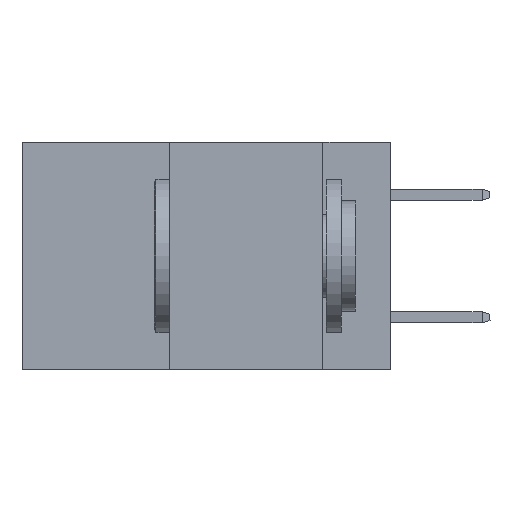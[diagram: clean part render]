
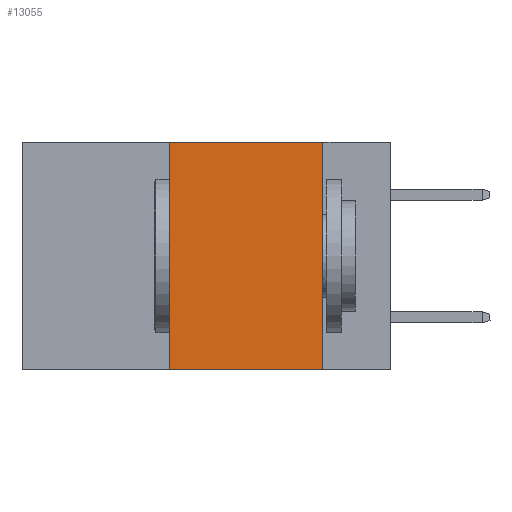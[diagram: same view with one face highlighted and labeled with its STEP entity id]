
A CAD part, left-side view. The second image highlights one B-rep face of the part: STEP entity #13055.
In plain terms, the highlighted planar face has unit normal (-1, 0, 0).
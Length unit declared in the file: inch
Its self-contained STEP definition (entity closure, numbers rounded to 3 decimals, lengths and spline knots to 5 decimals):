
#154 = LINE ( 'NONE', #2120, #3771 ) ;
#176 = DIRECTION ( 'NONE',  ( 0., 0., -1. ) ) ;
#605 = VERTEX_POINT ( 'NONE', #15817 ) ;
#864 = VECTOR ( 'NONE', #176, 39.37008 ) ;
#1067 = VERTEX_POINT ( 'NONE', #2170 ) ;
#2120 = CARTESIAN_POINT ( 'NONE',  ( 0., 0.6, 0. ) ) ;
#2170 = CARTESIAN_POINT ( 'NONE',  ( 0., 0.11, -0.37 ) ) ;
#2599 = VERTEX_POINT ( 'NONE', #12426 ) ;
#2916 = CARTESIAN_POINT ( 'NONE',  ( 0., 0.6, 0. ) ) ;
#3041 = DIRECTION ( 'NONE',  ( 0., 0., -1. ) ) ;
#3288 = LINE ( 'NONE', #18314, #15344 ) ;
#3771 = VECTOR ( 'NONE', #8255, 39.37008 ) ;
#3945 = ORIENTED_EDGE ( 'NONE', *, *, #11523, .F. ) ;
#4172 = DIRECTION ( 'NONE',  ( 0., -1., 0. ) ) ;
#4533 = EDGE_LOOP ( 'NONE', ( #7089, #3945, #11568, #16254 ) ) ;
#4848 = EDGE_CURVE ( 'NONE', #2599, #1067, #10076, .T. ) ;
#5058 = LINE ( 'NONE', #8774, #18072 ) ;
#7089 = ORIENTED_EDGE ( 'NONE', *, *, #4848, .F. ) ;
#8255 = DIRECTION ( 'NONE',  ( 0., -1., 0. ) ) ;
#8774 = CARTESIAN_POINT ( 'NONE',  ( 0., 0.6, -0.37 ) ) ;
#10076 = LINE ( 'NONE', #12621, #864 ) ;
#10418 = DIRECTION ( 'NONE',  ( 0., 0., 1. ) ) ;
#11523 = EDGE_CURVE ( 'NONE', #605, #2599, #154, .T. ) ;
#11568 = ORIENTED_EDGE ( 'NONE', *, *, #14917, .F. ) ;
#11653 = AXIS2_PLACEMENT_3D ( 'NONE', #2916, #12459, #3041 ) ;
#11708 = FACE_OUTER_BOUND ( 'NONE', #4533, .T. ) ;
#12426 = CARTESIAN_POINT ( 'NONE',  ( 0., 0.11, 0. ) ) ;
#12459 = DIRECTION ( 'NONE',  ( 1., 0., 0. ) ) ;
#12621 = CARTESIAN_POINT ( 'NONE',  ( 0., 0.11, 0. ) ) ;
#13055 = ADVANCED_FACE ( 'NONE', ( #11708 ), #18645, .F. ) ;
#14917 = EDGE_CURVE ( 'NONE', #20111, #605, #3288, .T. ) ;
#15344 = VECTOR ( 'NONE', #10418, 39.37008 ) ;
#15817 = CARTESIAN_POINT ( 'NONE',  ( 0., 0.36, 0. ) ) ;
#16091 = CARTESIAN_POINT ( 'NONE',  ( 0., 0.36, -0.37 ) ) ;
#16254 = ORIENTED_EDGE ( 'NONE', *, *, #18540, .T. ) ;
#18072 = VECTOR ( 'NONE', #4172, 39.37008 ) ;
#18314 = CARTESIAN_POINT ( 'NONE',  ( 0., 0.36, 0. ) ) ;
#18540 = EDGE_CURVE ( 'NONE', #20111, #1067, #5058, .T. ) ;
#18645 = PLANE ( 'NONE',  #11653 ) ;
#20111 = VERTEX_POINT ( 'NONE', #16091 ) ;
